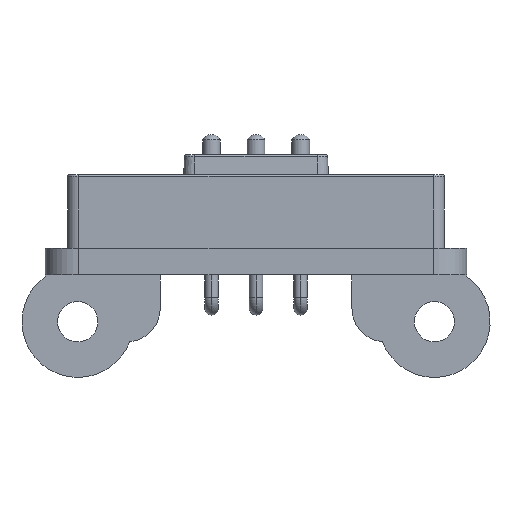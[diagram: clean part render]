
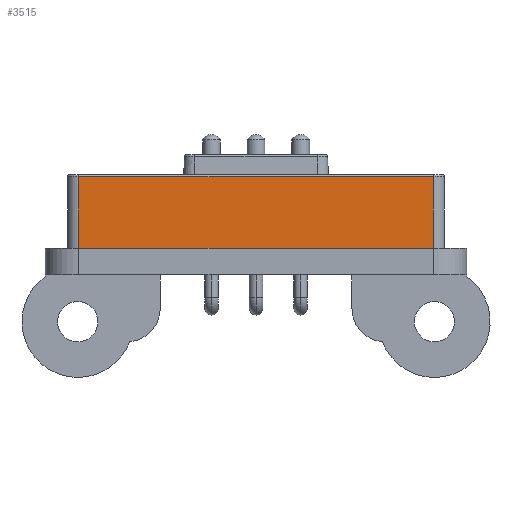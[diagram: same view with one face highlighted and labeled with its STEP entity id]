
A CAD part, front view. The second image highlights one B-rep face of the part: STEP entity #3515.
In plain terms, the highlighted planar face has unit normal (0, -1, 0).
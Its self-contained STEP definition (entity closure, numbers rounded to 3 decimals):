
#61 = VECTOR ( 'NONE', #2810, 1000. ) ;
#461 = DIRECTION ( 'NONE',  ( -1., 0., 0. ) ) ;
#467 = CARTESIAN_POINT ( 'NONE',  ( -7.95, -2., -3.3 ) ) ;
#468 = CARTESIAN_POINT ( 'NONE',  ( -7.95, -2., -0.1 ) ) ;
#603 = CARTESIAN_POINT ( 'NONE',  ( 7.95, -2., -3.3 ) ) ;
#606 = ORIENTED_EDGE ( 'NONE', *, *, #3594, .T. ) ;
#714 = VERTEX_POINT ( 'NONE', #467 ) ;
#851 = EDGE_CURVE ( 'NONE', #5328, #985, #5599, .T. ) ;
#910 = DIRECTION ( 'NONE',  ( 0., 1., 0. ) ) ;
#985 = VERTEX_POINT ( 'NONE', #4532 ) ;
#1303 = LINE ( 'NONE', #3516, #6755 ) ;
#1456 = FACE_OUTER_BOUND ( 'NONE', #2459, .T. ) ;
#1484 = ORIENTED_EDGE ( 'NONE', *, *, #1772, .T. ) ;
#1772 = EDGE_CURVE ( 'NONE', #714, #5328, #1303, .T. ) ;
#2289 = ORIENTED_EDGE ( 'NONE', *, *, #5700, .T. ) ;
#2459 = EDGE_LOOP ( 'NONE', ( #606, #1484, #3850, #2289 ) ) ;
#2672 = DIRECTION ( 'NONE',  ( 0., 0., -1. ) ) ;
#2810 = DIRECTION ( 'NONE',  ( 0., 0., 1. ) ) ;
#3125 = DIRECTION ( 'NONE',  ( 1., 0., 0. ) ) ;
#3130 = VECTOR ( 'NONE', #2672, 1000. ) ;
#3218 = LINE ( 'NONE', #5455, #6704 ) ;
#3515 = ADVANCED_FACE ( 'NONE', ( #1456 ), #3670, .F. ) ;
#3516 = CARTESIAN_POINT ( 'NONE',  ( -7.95, -2., -3.3 ) ) ;
#3594 = EDGE_CURVE ( 'NONE', #4320, #714, #5461, .T. ) ;
#3670 = PLANE ( 'NONE',  #4443 ) ;
#3850 = ORIENTED_EDGE ( 'NONE', *, *, #851, .T. ) ;
#4320 = VERTEX_POINT ( 'NONE', #6457 ) ;
#4443 = AXIS2_PLACEMENT_3D ( 'NONE', #5924, #910, #3125 ) ;
#4532 = CARTESIAN_POINT ( 'NONE',  ( 7.95, -2., -0.1 ) ) ;
#5328 = VERTEX_POINT ( 'NONE', #7217 ) ;
#5455 = CARTESIAN_POINT ( 'NONE',  ( 7.95, -2., -0.1 ) ) ;
#5461 = LINE ( 'NONE', #468, #3130 ) ;
#5599 = LINE ( 'NONE', #603, #61 ) ;
#5700 = EDGE_CURVE ( 'NONE', #985, #4320, #3218, .T. ) ;
#5763 = DIRECTION ( 'NONE',  ( 1., 0., 0. ) ) ;
#5924 = CARTESIAN_POINT ( 'NONE',  ( 0., -2., -1.7 ) ) ;
#6457 = CARTESIAN_POINT ( 'NONE',  ( -7.95, -2., -0.1 ) ) ;
#6704 = VECTOR ( 'NONE', #461, 1000. ) ;
#6755 = VECTOR ( 'NONE', #5763, 1000. ) ;
#7217 = CARTESIAN_POINT ( 'NONE',  ( 7.95, -2., -3.3 ) ) ;
